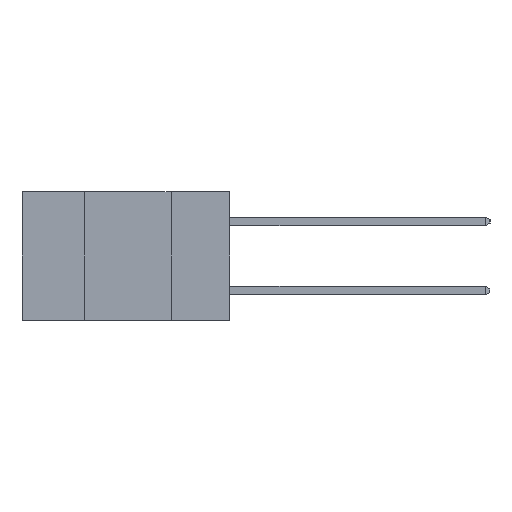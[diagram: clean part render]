
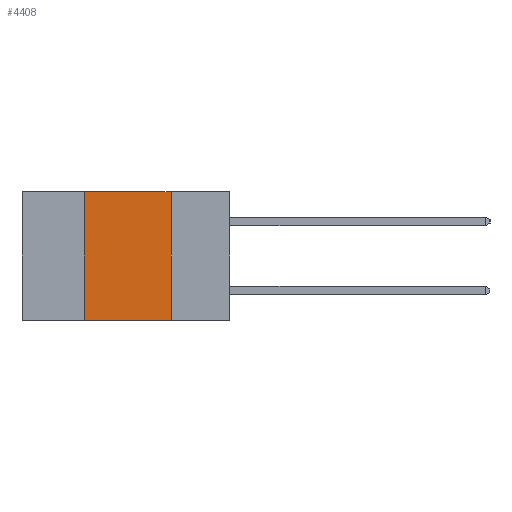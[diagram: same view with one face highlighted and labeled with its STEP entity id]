
A CAD part, left-side view. The second image highlights one B-rep face of the part: STEP entity #4408.
In plain terms, the highlighted planar face has unit normal (-1, 0, 0).
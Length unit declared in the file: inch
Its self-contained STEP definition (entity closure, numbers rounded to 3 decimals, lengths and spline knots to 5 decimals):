
#223 = DIRECTION ( 'NONE',  ( 0., 0., -1. ) ) ;
#320 = DIRECTION ( 'NONE',  ( 1., 0., 0. ) ) ;
#732 = DIRECTION ( 'NONE',  ( 0., -1., 0. ) ) ;
#784 = LINE ( 'NONE', #9714, #10601 ) ;
#1184 = EDGE_CURVE ( 'NONE', #3266, #8647, #12756, .T. ) ;
#1722 = LINE ( 'NONE', #6373, #4805 ) ;
#2859 = EDGE_CURVE ( 'NONE', #12469, #15709, #9560, .T. ) ;
#3200 = EDGE_CURVE ( 'NONE', #12469, #8647, #1722, .T. ) ;
#3266 = VERTEX_POINT ( 'NONE', #10724 ) ;
#4137 = FACE_OUTER_BOUND ( 'NONE', #11836, .T. ) ;
#4182 = DIRECTION ( 'NONE',  ( 0., 0., -1. ) ) ;
#4262 = CARTESIAN_POINT ( 'NONE',  ( 0., 0.17, 0. ) ) ;
#4408 = ADVANCED_FACE ( 'NONE', ( #4137 ), #14894, .F. ) ;
#4613 = AXIS2_PLACEMENT_3D ( 'NONE', #13475, #320, #223 ) ;
#4805 = VECTOR ( 'NONE', #12097, 39.37008 ) ;
#5389 = CARTESIAN_POINT ( 'NONE',  ( 0., 0.42, 0. ) ) ;
#5693 = CARTESIAN_POINT ( 'NONE',  ( 0., 0.42, 0. ) ) ;
#6120 = VECTOR ( 'NONE', #4182, 39.37008 ) ;
#6373 = CARTESIAN_POINT ( 'NONE',  ( 0., 0.6, -0.37 ) ) ;
#7447 = DIRECTION ( 'NONE',  ( 0., 0., 1. ) ) ;
#8647 = VERTEX_POINT ( 'NONE', #10793 ) ;
#9560 = LINE ( 'NONE', #5693, #12838 ) ;
#9714 = CARTESIAN_POINT ( 'NONE',  ( 0., 0.6, 0. ) ) ;
#9982 = EDGE_CURVE ( 'NONE', #15709, #3266, #784, .T. ) ;
#10601 = VECTOR ( 'NONE', #732, 39.37008 ) ;
#10724 = CARTESIAN_POINT ( 'NONE',  ( 0., 0.17, 0. ) ) ;
#10793 = CARTESIAN_POINT ( 'NONE',  ( 0., 0.17, -0.37 ) ) ;
#10827 = ORIENTED_EDGE ( 'NONE', *, *, #1184, .F. ) ;
#11224 = ORIENTED_EDGE ( 'NONE', *, *, #2859, .F. ) ;
#11522 = CARTESIAN_POINT ( 'NONE',  ( 0., 0.42, -0.37 ) ) ;
#11836 = EDGE_LOOP ( 'NONE', ( #10827, #14055, #11224, #14826 ) ) ;
#12097 = DIRECTION ( 'NONE',  ( 0., -1., 0. ) ) ;
#12469 = VERTEX_POINT ( 'NONE', #11522 ) ;
#12756 = LINE ( 'NONE', #4262, #6120 ) ;
#12838 = VECTOR ( 'NONE', #7447, 39.37008 ) ;
#13475 = CARTESIAN_POINT ( 'NONE',  ( 0., 0.6, 0. ) ) ;
#14055 = ORIENTED_EDGE ( 'NONE', *, *, #9982, .F. ) ;
#14826 = ORIENTED_EDGE ( 'NONE', *, *, #3200, .T. ) ;
#14894 = PLANE ( 'NONE',  #4613 ) ;
#15709 = VERTEX_POINT ( 'NONE', #5389 ) ;
